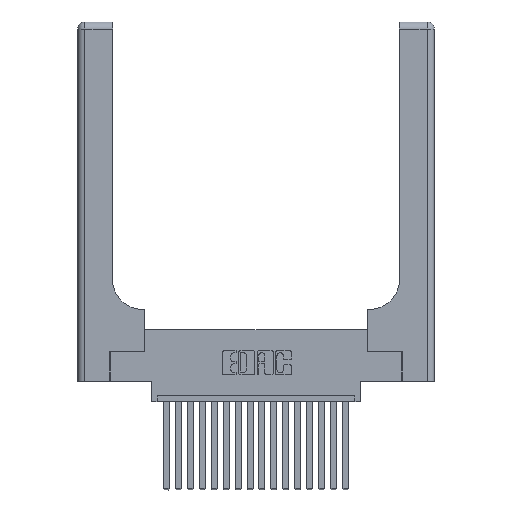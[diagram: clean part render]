
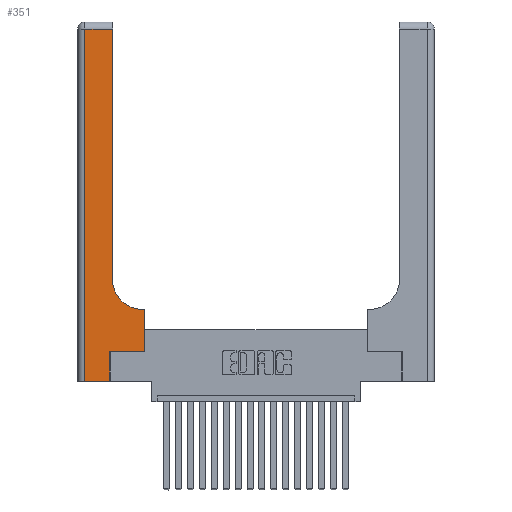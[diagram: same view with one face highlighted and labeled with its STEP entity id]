
A CAD part, top view. The second image highlights one B-rep face of the part: STEP entity #351.
In plain terms, the highlighted planar face has unit normal (0, 0, 1).
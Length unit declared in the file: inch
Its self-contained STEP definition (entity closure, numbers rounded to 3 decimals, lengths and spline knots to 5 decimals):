
#57 = CARTESIAN_POINT ( 'NONE',  ( 0.5585, 0.25, 0.37 ) ) ;
#101 = CARTESIAN_POINT ( 'NONE',  ( 0.5585, 0.6, 0.37 ) ) ;
#132 = VECTOR ( 'NONE', #8451, 39.37008 ) ;
#351 = ADVANCED_FACE ( 'NONE', ( #12297 ), #18537, .F. ) ;
#440 = CARTESIAN_POINT ( 'NONE',  ( 0.2915, 2.94, 0.37 ) ) ;
#517 = DIRECTION ( 'NONE',  ( 0., -1., 0. ) ) ;
#1370 = CARTESIAN_POINT ( 'NONE',  ( 0.269, 0.25, 0.37 ) ) ;
#1752 = DIRECTION ( 'NONE',  ( 1., 0., 0. ) ) ;
#2024 = DIRECTION ( 'NONE',  ( 1., 0., 0. ) ) ;
#2218 = CARTESIAN_POINT ( 'NONE',  ( 0.2915, 0.6, 0.37 ) ) ;
#2232 = ORIENTED_EDGE ( 'NONE', *, *, #2964, .T. ) ;
#2625 = VECTOR ( 'NONE', #1752, 39.37008 ) ;
#2701 = DIRECTION ( 'NONE',  ( 0., 1., 0. ) ) ;
#2964 = EDGE_CURVE ( 'NONE', #19871, #14129, #18047, .T. ) ;
#3404 = DIRECTION ( 'NONE',  ( 0., 1., 0. ) ) ;
#3414 = LINE ( 'NONE', #6827, #14651 ) ;
#3597 = ORIENTED_EDGE ( 'NONE', *, *, #14488, .T. ) ;
#3671 = LINE ( 'NONE', #2218, #132 ) ;
#3769 = DIRECTION ( 'NONE',  ( 1., 0., 0. ) ) ;
#3865 = LINE ( 'NONE', #11316, #2625 ) ;
#3975 = VECTOR ( 'NONE', #3404, 39.37008 ) ;
#4016 = CARTESIAN_POINT ( 'NONE',  ( 0., 2.94, 0.37 ) ) ;
#5820 = VECTOR ( 'NONE', #517, 39.37008 ) ;
#5952 = CARTESIAN_POINT ( 'NONE',  ( 0.2915, 3., 0.37 ) ) ;
#6110 = VERTEX_POINT ( 'NONE', #440 ) ;
#6112 = VERTEX_POINT ( 'NONE', #15119 ) ;
#6327 = EDGE_LOOP ( 'NONE', ( #6446, #14251, #2232, #8256, #8239, #17259, #3597, #20689, #8422 ) ) ;
#6446 = ORIENTED_EDGE ( 'NONE', *, *, #18916, .T. ) ;
#6503 = CARTESIAN_POINT ( 'NONE',  ( 0.5585, 0.25, 0.37 ) ) ;
#6827 = CARTESIAN_POINT ( 'NONE',  ( 0., 0., 0.37 ) ) ;
#7283 = VERTEX_POINT ( 'NONE', #57 ) ;
#8239 = ORIENTED_EDGE ( 'NONE', *, *, #10609, .T. ) ;
#8256 = ORIENTED_EDGE ( 'NONE', *, *, #9471, .T. ) ;
#8382 = DIRECTION ( 'NONE',  ( 0., 0., -1. ) ) ;
#8422 = ORIENTED_EDGE ( 'NONE', *, *, #11820, .T. ) ;
#8451 = DIRECTION ( 'NONE',  ( -1., 0., 0. ) ) ;
#9143 = CARTESIAN_POINT ( 'NONE',  ( 0., 3., 0.37 ) ) ;
#9471 = EDGE_CURVE ( 'NONE', #14129, #10576, #3414, .T. ) ;
#10576 = VERTEX_POINT ( 'NONE', #14421 ) ;
#10609 = EDGE_CURVE ( 'NONE', #10576, #20280, #18063, .T. ) ;
#10765 = DIRECTION ( 'NONE',  ( 0., 0., -1. ) ) ;
#11215 = CARTESIAN_POINT ( 'NONE',  ( 0.06, 2.94, 0.37 ) ) ;
#11316 = CARTESIAN_POINT ( 'NONE',  ( 0.269, 0.25, 0.37 ) ) ;
#11537 = CARTESIAN_POINT ( 'NONE',  ( 0.06, 0., 0.37 ) ) ;
#11820 = EDGE_CURVE ( 'NONE', #15345, #6112, #13326, .T. ) ;
#12192 = AXIS2_PLACEMENT_3D ( 'NONE', #16459, #8382, #2024 ) ;
#12297 = FACE_OUTER_BOUND ( 'NONE', #6327, .T. ) ;
#13163 = EDGE_CURVE ( 'NONE', #6110, #19871, #14498, .T. ) ;
#13186 = DIRECTION ( 'NONE',  ( 0., 1., 0. ) ) ;
#13317 = CARTESIAN_POINT ( 'NONE',  ( 0.269, 0., 0.37 ) ) ;
#13326 = CIRCLE ( 'NONE', #12192, 0.25 ) ;
#13396 = VECTOR ( 'NONE', #2701, 39.37008 ) ;
#13959 = VERTEX_POINT ( 'NONE', #101 ) ;
#14129 = VERTEX_POINT ( 'NONE', #11537 ) ;
#14247 = VECTOR ( 'NONE', #18357, 39.37008 ) ;
#14251 = ORIENTED_EDGE ( 'NONE', *, *, #13163, .T. ) ;
#14421 = CARTESIAN_POINT ( 'NONE',  ( 0.269, 0., 0.37 ) ) ;
#14488 = EDGE_CURVE ( 'NONE', #7283, #13959, #20664, .T. ) ;
#14498 = LINE ( 'NONE', #4016, #14247 ) ;
#14651 = VECTOR ( 'NONE', #3769, 39.37008 ) ;
#15119 = CARTESIAN_POINT ( 'NONE',  ( 0.2915, 0.85, 0.37 ) ) ;
#15345 = VERTEX_POINT ( 'NONE', #18405 ) ;
#16176 = CARTESIAN_POINT ( 'NONE',  ( 0.06, 3., 0.37 ) ) ;
#16459 = CARTESIAN_POINT ( 'NONE',  ( 0.5415, 0.85, 0.37 ) ) ;
#17259 = ORIENTED_EDGE ( 'NONE', *, *, #19766, .T. ) ;
#17546 = VECTOR ( 'NONE', #13186, 39.37008 ) ;
#18047 = LINE ( 'NONE', #16176, #5820 ) ;
#18063 = LINE ( 'NONE', #13317, #17546 ) ;
#18357 = DIRECTION ( 'NONE',  ( -1., 0., 0. ) ) ;
#18405 = CARTESIAN_POINT ( 'NONE',  ( 0.5415, 0.6, 0.37 ) ) ;
#18537 = PLANE ( 'NONE',  #19515 ) ;
#18614 = EDGE_CURVE ( 'NONE', #13959, #15345, #3671, .T. ) ;
#18862 = LINE ( 'NONE', #5952, #13396 ) ;
#18916 = EDGE_CURVE ( 'NONE', #6112, #6110, #18862, .T. ) ;
#19515 = AXIS2_PLACEMENT_3D ( 'NONE', #9143, #10765, #20120 ) ;
#19766 = EDGE_CURVE ( 'NONE', #20280, #7283, #3865, .T. ) ;
#19871 = VERTEX_POINT ( 'NONE', #11215 ) ;
#20120 = DIRECTION ( 'NONE',  ( -1., 0., 0. ) ) ;
#20280 = VERTEX_POINT ( 'NONE', #1370 ) ;
#20664 = LINE ( 'NONE', #6503, #3975 ) ;
#20689 = ORIENTED_EDGE ( 'NONE', *, *, #18614, .T. ) ;
